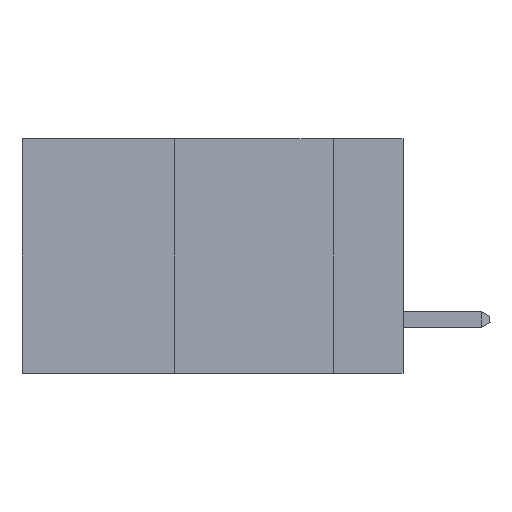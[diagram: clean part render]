
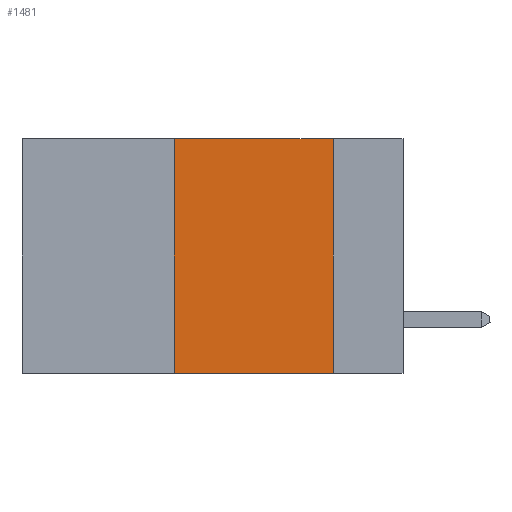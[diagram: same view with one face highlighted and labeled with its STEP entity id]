
A CAD part, left-side view. The second image highlights one B-rep face of the part: STEP entity #1481.
In plain terms, the highlighted planar face has unit normal (-1, 0, 0).
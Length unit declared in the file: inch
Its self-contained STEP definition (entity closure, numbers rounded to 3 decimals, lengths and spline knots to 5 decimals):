
#1409 = CARTESIAN_POINT ( 'NONE',  ( 0., 0.6, 0. ) ) ;
#1481 = ADVANCED_FACE ( 'NONE', ( #1987 ), #14721, .F. ) ;
#1719 = VERTEX_POINT ( 'NONE', #14748 ) ;
#1894 = DIRECTION ( 'NONE',  ( 0., 0., -1. ) ) ;
#1965 = VECTOR ( 'NONE', #23671, 39.37008 ) ;
#1987 = FACE_OUTER_BOUND ( 'NONE', #2721, .T. ) ;
#2721 = EDGE_LOOP ( 'NONE', ( #13342, #10324, #21246, #17876 ) ) ;
#4011 = DIRECTION ( 'NONE',  ( 0., 0., 1. ) ) ;
#5932 = CARTESIAN_POINT ( 'NONE',  ( 0., 0.36, 0. ) ) ;
#6207 = LINE ( 'NONE', #8850, #15735 ) ;
#6979 = CARTESIAN_POINT ( 'NONE',  ( 0., 0.11, -0.37 ) ) ;
#7310 = VERTEX_POINT ( 'NONE', #10374 ) ;
#7931 = CARTESIAN_POINT ( 'NONE',  ( 0., 0.11, 0. ) ) ;
#8120 = LINE ( 'NONE', #5932, #13520 ) ;
#8581 = VERTEX_POINT ( 'NONE', #6979 ) ;
#8850 = CARTESIAN_POINT ( 'NONE',  ( 0., 0.6, -0.37 ) ) ;
#10324 = ORIENTED_EDGE ( 'NONE', *, *, #11951, .F. ) ;
#10374 = CARTESIAN_POINT ( 'NONE',  ( 0., 0.36, 0. ) ) ;
#11392 = AXIS2_PLACEMENT_3D ( 'NONE', #12734, #24237, #1894 ) ;
#11951 = EDGE_CURVE ( 'NONE', #7310, #23267, #12729, .T. ) ;
#12342 = LINE ( 'NONE', #20887, #18674 ) ;
#12729 = LINE ( 'NONE', #1409, #1965 ) ;
#12734 = CARTESIAN_POINT ( 'NONE',  ( 0., 0.6, 0. ) ) ;
#13342 = ORIENTED_EDGE ( 'NONE', *, *, #18739, .F. ) ;
#13520 = VECTOR ( 'NONE', #4011, 39.37008 ) ;
#14174 = EDGE_CURVE ( 'NONE', #1719, #8581, #6207, .T. ) ;
#14721 = PLANE ( 'NONE',  #11392 ) ;
#14748 = CARTESIAN_POINT ( 'NONE',  ( 0., 0.36, -0.37 ) ) ;
#15735 = VECTOR ( 'NONE', #24972, 39.37008 ) ;
#17876 = ORIENTED_EDGE ( 'NONE', *, *, #14174, .T. ) ;
#18674 = VECTOR ( 'NONE', #24754, 39.37008 ) ;
#18739 = EDGE_CURVE ( 'NONE', #23267, #8581, #12342, .T. ) ;
#20887 = CARTESIAN_POINT ( 'NONE',  ( 0., 0.11, 0. ) ) ;
#21246 = ORIENTED_EDGE ( 'NONE', *, *, #26049, .F. ) ;
#23267 = VERTEX_POINT ( 'NONE', #7931 ) ;
#23671 = DIRECTION ( 'NONE',  ( 0., -1., 0. ) ) ;
#24237 = DIRECTION ( 'NONE',  ( 1., 0., 0. ) ) ;
#24754 = DIRECTION ( 'NONE',  ( 0., 0., -1. ) ) ;
#24972 = DIRECTION ( 'NONE',  ( 0., -1., 0. ) ) ;
#26049 = EDGE_CURVE ( 'NONE', #1719, #7310, #8120, .T. ) ;
